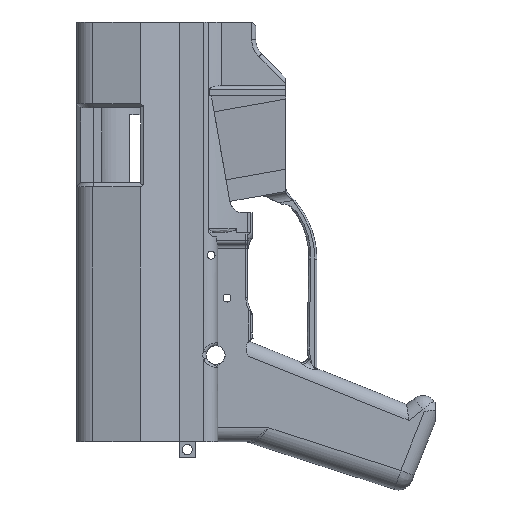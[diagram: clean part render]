
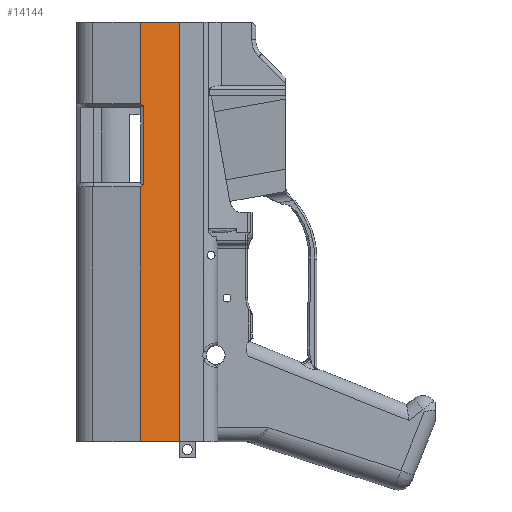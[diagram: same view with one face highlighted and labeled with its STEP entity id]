
A CAD part, left-side view. The second image highlights one B-rep face of the part: STEP entity #14144.
In plain terms, the highlighted planar face has unit normal (-0.954, -0.299, 0).
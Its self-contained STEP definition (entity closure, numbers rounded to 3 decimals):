
#390 = VERTEX_POINT ( 'NONE', #5320 ) ;
#541 = PLANE ( 'NONE',  #11332 ) ;
#598 = LINE ( 'NONE', #3011, #2067 ) ;
#974 = ORIENTED_EDGE ( 'NONE', *, *, #14075, .F. ) ;
#1123 = VERTEX_POINT ( 'NONE', #6166 ) ;
#1200 = CARTESIAN_POINT ( 'NONE',  ( -11.97, 67.065, 120.735 ) ) ;
#1529 = VERTEX_POINT ( 'NONE', #7033 ) ;
#1801 = DIRECTION ( 'NONE',  ( -0.299, 0.954, 0. ) ) ;
#1821 = LINE ( 'NONE', #8862, #2555 ) ;
#1910 = ORIENTED_EDGE ( 'NONE', *, *, #2805, .F. ) ;
#1933 = CARTESIAN_POINT ( 'NONE',  ( -5.851, 47.507, 120.735 ) ) ;
#1982 = DIRECTION ( 'NONE',  ( 0., 0., 1. ) ) ;
#2067 = VECTOR ( 'NONE', #7714, 1000. ) ;
#2079 = CARTESIAN_POINT ( 'NONE',  ( -18.446, 87.767, 299.852 ) ) ;
#2141 = DIRECTION ( 'NONE',  ( 0.27, -0.862, -0.428 ) ) ;
#2555 = VECTOR ( 'NONE', #1801, 1000. ) ;
#2738 = EDGE_CURVE ( 'NONE', #8922, #8292, #1821, .T. ) ;
#2805 = EDGE_CURVE ( 'NONE', #1123, #11734, #3293, .T. ) ;
#2918 = CARTESIAN_POINT ( 'NONE',  ( 8.207, 2.568, 158.835 ) ) ;
#3011 = CARTESIAN_POINT ( 'NONE',  ( -11.97, 67.065, 158.835 ) ) ;
#3233 = EDGE_CURVE ( 'NONE', #7519, #1123, #9150, .T. ) ;
#3293 = LINE ( 'NONE', #12264, #10769 ) ;
#3741 = DIRECTION ( 'NONE',  ( -0.27, 0.862, -0.428 ) ) ;
#4302 = VECTOR ( 'NONE', #10244, 1000. ) ;
#4334 = CARTESIAN_POINT ( 'NONE',  ( -5.851, 47.507, 158.835 ) ) ;
#4354 = CARTESIAN_POINT ( 'NONE',  ( -11.372, 65.157, 158.835 ) ) ;
#4672 = LINE ( 'NONE', #4354, #4302 ) ;
#5320 = CARTESIAN_POINT ( 'NONE',  ( -11.372, 65.157, 288.626 ) ) ;
#5347 = ORIENTED_EDGE ( 'NONE', *, *, #8823, .T. ) ;
#5717 = VECTOR ( 'NONE', #3741, 1000. ) ;
#5991 = EDGE_CURVE ( 'NONE', #390, #1529, #4672, .T. ) ;
#6129 = CARTESIAN_POINT ( 'NONE',  ( -11.97, 67.065, 158.835 ) ) ;
#6166 = CARTESIAN_POINT ( 'NONE',  ( -11.97, 67.065, 330.482 ) ) ;
#7033 = CARTESIAN_POINT ( 'NONE',  ( -11.372, 65.157, 249.118 ) ) ;
#7264 = ORIENTED_EDGE ( 'NONE', *, *, #2738, .F. ) ;
#7519 = VERTEX_POINT ( 'NONE', #10964 ) ;
#7526 = ORIENTED_EDGE ( 'NONE', *, *, #5991, .T. ) ;
#7634 = VERTEX_POINT ( 'NONE', #7667 ) ;
#7667 = CARTESIAN_POINT ( 'NONE',  ( -11.97, 67.065, 248.171 ) ) ;
#7714 = DIRECTION ( 'NONE',  ( 0., 0., 1. ) ) ;
#8292 = VERTEX_POINT ( 'NONE', #1200 ) ;
#8493 = LINE ( 'NONE', #4334, #12696 ) ;
#8605 = DIRECTION ( 'NONE',  ( 0., 0., 1. ) ) ;
#8823 = EDGE_CURVE ( 'NONE', #8922, #11734, #8493, .T. ) ;
#8862 = CARTESIAN_POINT ( 'NONE',  ( 8.207, 2.568, 120.735 ) ) ;
#8922 = VERTEX_POINT ( 'NONE', #1933 ) ;
#9044 = FACE_OUTER_BOUND ( 'NONE', #9848, .T. ) ;
#9130 = CARTESIAN_POINT ( 'NONE',  ( -5.851, 47.507, 330.482 ) ) ;
#9150 = LINE ( 'NONE', #6129, #10944 ) ;
#9396 = LINE ( 'NONE', #2079, #11743 ) ;
#9423 = ORIENTED_EDGE ( 'NONE', *, *, #3233, .F. ) ;
#9605 = EDGE_CURVE ( 'NONE', #1529, #7634, #11927, .T. ) ;
#9848 = EDGE_LOOP ( 'NONE', ( #9423, #11587, #7526, #10527, #974, #7264, #5347, #1910 ) ) ;
#10244 = DIRECTION ( 'NONE',  ( 0., 0., -1. ) ) ;
#10527 = ORIENTED_EDGE ( 'NONE', *, *, #9605, .T. ) ;
#10635 = CARTESIAN_POINT ( 'NONE',  ( -18.446, 87.767, 237.892 ) ) ;
#10769 = VECTOR ( 'NONE', #12317, 1000. ) ;
#10944 = VECTOR ( 'NONE', #8605, 1000. ) ;
#10964 = CARTESIAN_POINT ( 'NONE',  ( -11.97, 67.065, 289.574 ) ) ;
#11332 = AXIS2_PLACEMENT_3D ( 'NONE', #2918, #13653, #13756 ) ;
#11587 = ORIENTED_EDGE ( 'NONE', *, *, #14215, .T. ) ;
#11734 = VERTEX_POINT ( 'NONE', #9130 ) ;
#11743 = VECTOR ( 'NONE', #2141, 1000. ) ;
#11927 = LINE ( 'NONE', #10635, #5717 ) ;
#12264 = CARTESIAN_POINT ( 'NONE',  ( 8.207, 2.568, 330.482 ) ) ;
#12317 = DIRECTION ( 'NONE',  ( 0.299, -0.954, 0. ) ) ;
#12696 = VECTOR ( 'NONE', #1982, 1000. ) ;
#13653 = DIRECTION ( 'NONE',  ( 0.954, 0.299, 0. ) ) ;
#13756 = DIRECTION ( 'NONE',  ( -0.299, 0.954, 0. ) ) ;
#14075 = EDGE_CURVE ( 'NONE', #8292, #7634, #598, .T. ) ;
#14144 = ADVANCED_FACE ( 'NONE', ( #9044 ), #541, .F. ) ;
#14215 = EDGE_CURVE ( 'NONE', #7519, #390, #9396, .T. ) ;
